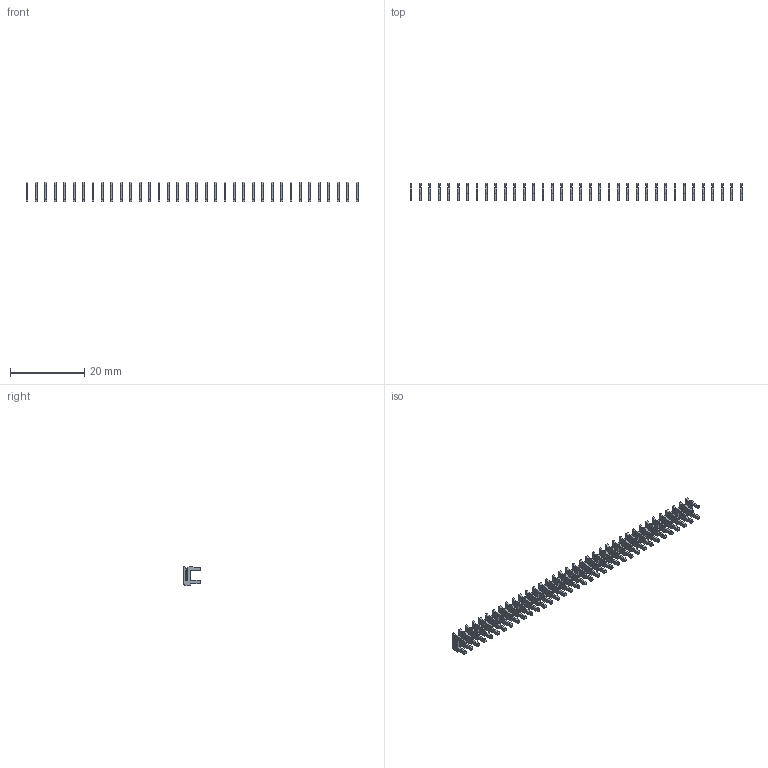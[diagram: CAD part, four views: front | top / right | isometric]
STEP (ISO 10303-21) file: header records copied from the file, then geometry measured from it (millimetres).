
FILE_DESCRIPTION (( 'STEP AP203' ), '1' );
FILE_NAME ('105-036-208-100.STEP', '2020-04-07T23:45:18', ( '' ), ( '' ), 'SwSTEP 2.0', 'SolidWorks 2016', '' );
FILE_SCHEMA (( 'CONFIG_CONTROL_DESIGN' ));
Length unit declared in the file: inch
Products named in the file (2): 100-290-001_100-290-208; 105-036-208-100
Assembly tree (36 placements, depth 2):
  105-036-208-100
    100-290-001_100-290-208  x36
Bounding box: 89.41 x 4.83 x 5.17 mm (x, y, z)
Volume: 247.7 mm3; surface area: 1529.9 mm2
Topology: 36 solids, 36 shells, 900 faces, 2484 edges, 1656 vertices
Faces by surface type: plane 792, cylinder 108
Entity records: 2109 total; most frequent: DIRECTION 203, CARTESIAN_POINT 179, ORIENTED_EDGE 138, LOCAL_TIME 82, CALENDAR_DATE 82, COORDINATED_UNIVERSAL_TIME_OFFSET 82, DATE_AND_TIME 82, AXIS2_PLACEMENT_3D 70
